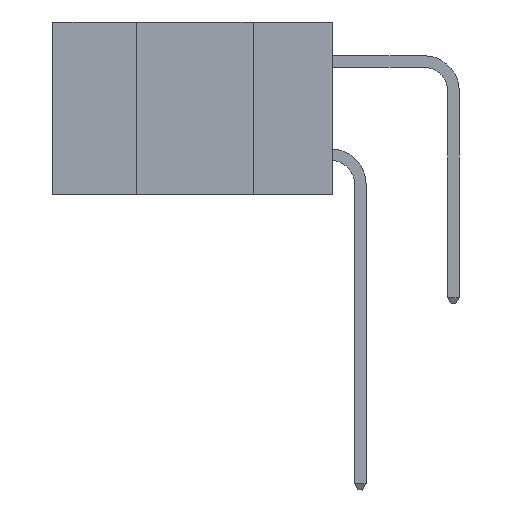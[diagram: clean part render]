
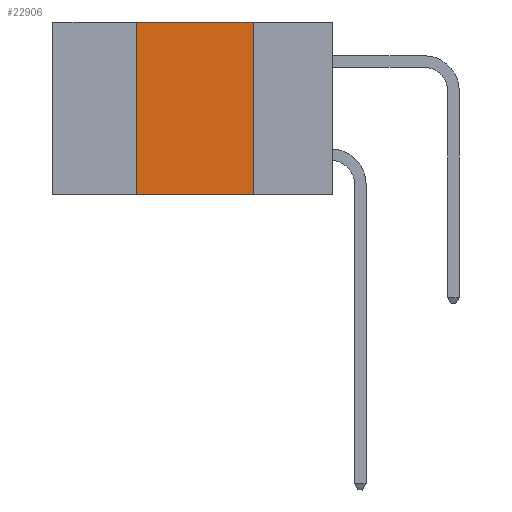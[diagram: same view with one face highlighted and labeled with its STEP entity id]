
A CAD part, left-side view. The second image highlights one B-rep face of the part: STEP entity #22906.
In plain terms, the highlighted planar face has unit normal (-1, 0, 0).
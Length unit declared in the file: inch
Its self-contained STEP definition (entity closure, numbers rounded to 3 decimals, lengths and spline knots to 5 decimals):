
#1435 = VECTOR ( 'NONE', #3241, 39.37008 ) ;
#1815 = LINE ( 'NONE', #21930, #1435 ) ;
#1838 = VECTOR ( 'NONE', #25516, 39.37008 ) ;
#3241 = DIRECTION ( 'NONE',  ( 0., -1., 0. ) ) ;
#3706 = VERTEX_POINT ( 'NONE', #10853 ) ;
#4158 = VECTOR ( 'NONE', #16812, 39.37008 ) ;
#5853 = EDGE_CURVE ( 'NONE', #3706, #12873, #17412, .T. ) ;
#6617 = EDGE_CURVE ( 'NONE', #19323, #6624, #7467, .T. ) ;
#6624 = VERTEX_POINT ( 'NONE', #10958 ) ;
#7134 = PLANE ( 'NONE',  #21282 ) ;
#7467 = LINE ( 'NONE', #11055, #24707 ) ;
#10853 = CARTESIAN_POINT ( 'NONE',  ( 0., 0.42, -0.37 ) ) ;
#10958 = CARTESIAN_POINT ( 'NONE',  ( 0., 0.17, -0.37 ) ) ;
#11013 = EDGE_CURVE ( 'NONE', #3706, #6624, #1815, .T. ) ;
#11055 = CARTESIAN_POINT ( 'NONE',  ( 0., 0.17, 0. ) ) ;
#12233 = LINE ( 'NONE', #16108, #1838 ) ;
#12873 = VERTEX_POINT ( 'NONE', #30199 ) ;
#14086 = DIRECTION ( 'NONE',  ( 1., 0., 0. ) ) ;
#15110 = ORIENTED_EDGE ( 'NONE', *, *, #16532, .F. ) ;
#16108 = CARTESIAN_POINT ( 'NONE',  ( 0., 0.6, 0. ) ) ;
#16532 = EDGE_CURVE ( 'NONE', #12873, #19323, #12233, .T. ) ;
#16812 = DIRECTION ( 'NONE',  ( 0., 0., 1. ) ) ;
#17220 = EDGE_LOOP ( 'NONE', ( #23015, #15110, #21461, #18430 ) ) ;
#17412 = LINE ( 'NONE', #23879, #4158 ) ;
#18430 = ORIENTED_EDGE ( 'NONE', *, *, #11013, .T. ) ;
#19087 = CARTESIAN_POINT ( 'NONE',  ( 0., 0.6, 0. ) ) ;
#19323 = VERTEX_POINT ( 'NONE', #29211 ) ;
#21282 = AXIS2_PLACEMENT_3D ( 'NONE', #19087, #14086, #25748 ) ;
#21461 = ORIENTED_EDGE ( 'NONE', *, *, #5853, .F. ) ;
#21930 = CARTESIAN_POINT ( 'NONE',  ( 0., 0.6, -0.37 ) ) ;
#22875 = DIRECTION ( 'NONE',  ( 0., 0., -1. ) ) ;
#22906 = ADVANCED_FACE ( 'NONE', ( #25890 ), #7134, .F. ) ;
#23015 = ORIENTED_EDGE ( 'NONE', *, *, #6617, .F. ) ;
#23879 = CARTESIAN_POINT ( 'NONE',  ( 0., 0.42, 0. ) ) ;
#24707 = VECTOR ( 'NONE', #22875, 39.37008 ) ;
#25516 = DIRECTION ( 'NONE',  ( 0., -1., 0. ) ) ;
#25748 = DIRECTION ( 'NONE',  ( 0., 0., -1. ) ) ;
#25890 = FACE_OUTER_BOUND ( 'NONE', #17220, .T. ) ;
#29211 = CARTESIAN_POINT ( 'NONE',  ( 0., 0.17, 0. ) ) ;
#30199 = CARTESIAN_POINT ( 'NONE',  ( 0., 0.42, 0. ) ) ;
